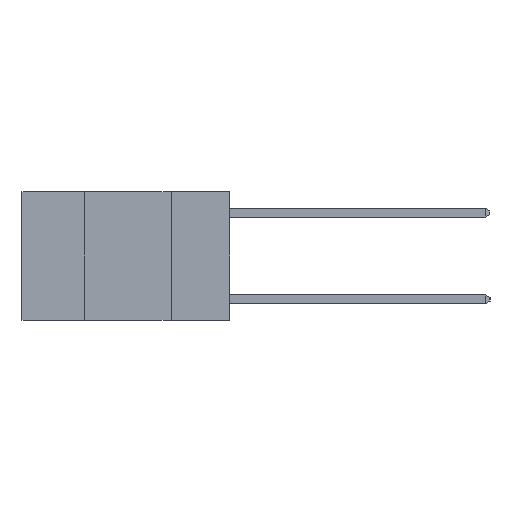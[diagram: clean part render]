
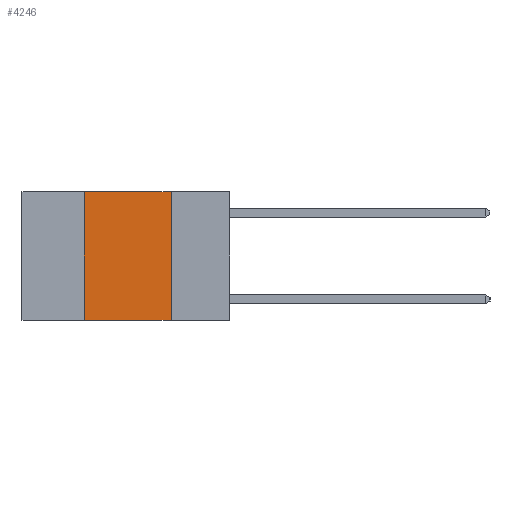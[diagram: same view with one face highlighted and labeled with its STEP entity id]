
A CAD part, left-side view. The second image highlights one B-rep face of the part: STEP entity #4246.
In plain terms, the highlighted planar face has unit normal (-1, 0, 0).
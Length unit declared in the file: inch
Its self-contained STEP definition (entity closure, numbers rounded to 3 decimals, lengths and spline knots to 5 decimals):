
#460 = CARTESIAN_POINT ( 'NONE',  ( 0., 0.42, -0.37 ) ) ;
#916 = CARTESIAN_POINT ( 'NONE',  ( 0., 0.42, 0. ) ) ;
#920 = LINE ( 'NONE', #5552, #2919 ) ;
#1380 = CARTESIAN_POINT ( 'NONE',  ( 0., 0.6, 0. ) ) ;
#1561 = DIRECTION ( 'NONE',  ( 0., -1., 0. ) ) ;
#1984 = LINE ( 'NONE', #916, #3554 ) ;
#2329 = PLANE ( 'NONE',  #5900 ) ;
#2530 = EDGE_CURVE ( 'NONE', #6460, #5108, #1984, .T. ) ;
#2573 = EDGE_CURVE ( 'NONE', #5054, #3913, #6733, .T. ) ;
#2919 = VECTOR ( 'NONE', #1561, 39.37008 ) ;
#3001 = DIRECTION ( 'NONE',  ( 1., 0., 0. ) ) ;
#3083 = EDGE_CURVE ( 'NONE', #6460, #3913, #920, .T. ) ;
#3154 = VECTOR ( 'NONE', #5662, 39.37008 ) ;
#3319 = CARTESIAN_POINT ( 'NONE',  ( 0., 0.42, 0. ) ) ;
#3401 = ORIENTED_EDGE ( 'NONE', *, *, #2530, .F. ) ;
#3554 = VECTOR ( 'NONE', #4275, 39.37008 ) ;
#3913 = VERTEX_POINT ( 'NONE', #5239 ) ;
#4017 = FACE_OUTER_BOUND ( 'NONE', #7615, .T. ) ;
#4056 = DIRECTION ( 'NONE',  ( 0., -1., 0. ) ) ;
#4092 = EDGE_CURVE ( 'NONE', #5108, #5054, #7156, .T. ) ;
#4246 = ADVANCED_FACE ( 'NONE', ( #4017 ), #2329, .F. ) ;
#4275 = DIRECTION ( 'NONE',  ( 0., 0., 1. ) ) ;
#4953 = CARTESIAN_POINT ( 'NONE',  ( 0., 0.17, 0. ) ) ;
#5054 = VERTEX_POINT ( 'NONE', #8026 ) ;
#5108 = VERTEX_POINT ( 'NONE', #3319 ) ;
#5239 = CARTESIAN_POINT ( 'NONE',  ( 0., 0.17, -0.37 ) ) ;
#5281 = VECTOR ( 'NONE', #4056, 39.37008 ) ;
#5552 = CARTESIAN_POINT ( 'NONE',  ( 0., 0.6, -0.37 ) ) ;
#5662 = DIRECTION ( 'NONE',  ( 0., 0., -1. ) ) ;
#5737 = ORIENTED_EDGE ( 'NONE', *, *, #2573, .F. ) ;
#5900 = AXIS2_PLACEMENT_3D ( 'NONE', #8374, #3001, #7728 ) ;
#6460 = VERTEX_POINT ( 'NONE', #460 ) ;
#6651 = ORIENTED_EDGE ( 'NONE', *, *, #4092, .F. ) ;
#6733 = LINE ( 'NONE', #4953, #3154 ) ;
#7156 = LINE ( 'NONE', #1380, #5281 ) ;
#7326 = ORIENTED_EDGE ( 'NONE', *, *, #3083, .T. ) ;
#7615 = EDGE_LOOP ( 'NONE', ( #5737, #6651, #3401, #7326 ) ) ;
#7728 = DIRECTION ( 'NONE',  ( 0., 0., -1. ) ) ;
#8026 = CARTESIAN_POINT ( 'NONE',  ( 0., 0.17, 0. ) ) ;
#8374 = CARTESIAN_POINT ( 'NONE',  ( 0., 0.6, 0. ) ) ;
